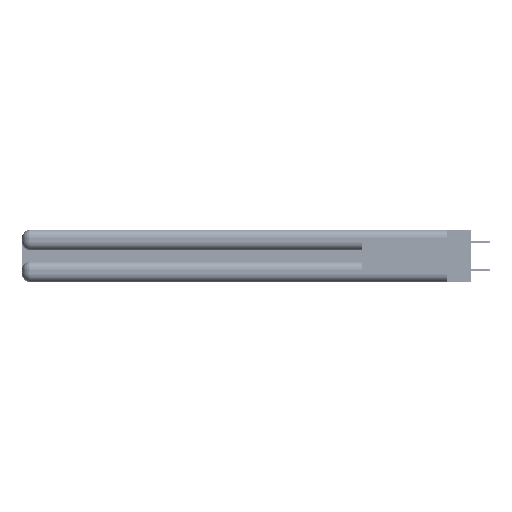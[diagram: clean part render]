
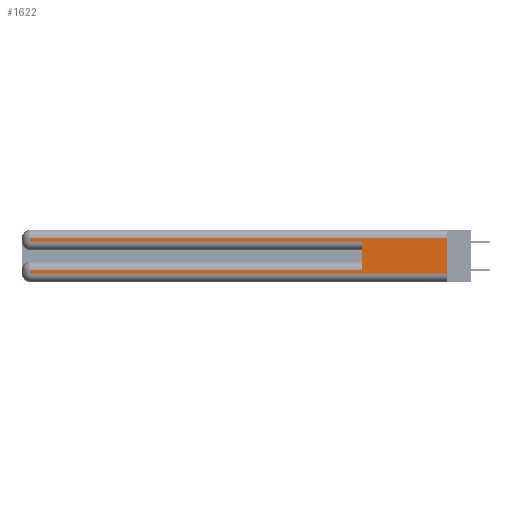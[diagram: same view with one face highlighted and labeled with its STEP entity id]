
A CAD part, left-side view. The second image highlights one B-rep face of the part: STEP entity #1622.
In plain terms, the highlighted planar face has unit normal (-1, 0, 0).
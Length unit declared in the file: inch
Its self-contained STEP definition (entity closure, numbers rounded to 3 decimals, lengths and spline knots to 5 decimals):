
#1622 = ADVANCED_FACE ( 'NONE', ( #33654 ), #19907, .F. ) ;
#1812 = CARTESIAN_POINT ( 'NONE',  ( 0., 2.94, 0.085 ) ) ;
#1971 = VERTEX_POINT ( 'NONE', #1812 ) ;
#2224 = DIRECTION ( 'NONE',  ( 0., -1., 0. ) ) ;
#2310 = ORIENTED_EDGE ( 'NONE', *, *, #7565, .T. ) ;
#2931 = ORIENTED_EDGE ( 'NONE', *, *, #28584, .F. ) ;
#3333 = CARTESIAN_POINT ( 'NONE',  ( 0., 2.94, 0.06 ) ) ;
#4153 = CARTESIAN_POINT ( 'NONE',  ( 0., 0.6, 0.085 ) ) ;
#4446 = CARTESIAN_POINT ( 'NONE',  ( 0., 0., 0.31 ) ) ;
#5204 = LINE ( 'NONE', #13782, #29299 ) ;
#5914 = ORIENTED_EDGE ( 'NONE', *, *, #37096, .T. ) ;
#6305 = VERTEX_POINT ( 'NONE', #4153 ) ;
#6535 = EDGE_CURVE ( 'NONE', #6305, #12182, #52799, .T. ) ;
#7017 = CARTESIAN_POINT ( 'NONE',  ( 0., 0., 0.37 ) ) ;
#7446 = VERTEX_POINT ( 'NONE', #29371 ) ;
#7565 = EDGE_CURVE ( 'NONE', #7446, #44319, #13025, .T. ) ;
#7586 = DIRECTION ( 'NONE',  ( 0., 0., -1. ) ) ;
#7832 = VECTOR ( 'NONE', #31057, 39.37008 ) ;
#11107 = LINE ( 'NONE', #50042, #44562 ) ;
#12182 = VERTEX_POINT ( 'NONE', #29759 ) ;
#13025 = LINE ( 'NONE', #4446, #52068 ) ;
#13201 = CARTESIAN_POINT ( 'NONE',  ( 0., 0., 0.37 ) ) ;
#13220 = DIRECTION ( 'NONE',  ( 0., -1., 0. ) ) ;
#13572 = CARTESIAN_POINT ( 'NONE',  ( 0., 0.6, 0.145 ) ) ;
#13758 = DIRECTION ( 'NONE',  ( 0., 0., -1. ) ) ;
#13782 = CARTESIAN_POINT ( 'NONE',  ( 0., 0., 0.285 ) ) ;
#13937 = VECTOR ( 'NONE', #32113, 39.37008 ) ;
#14042 = LINE ( 'NONE', #13201, #56431 ) ;
#17269 = DIRECTION ( 'NONE',  ( 0., 1., 0. ) ) ;
#17518 = EDGE_CURVE ( 'NONE', #6305, #1971, #34457, .T. ) ;
#19554 = VERTEX_POINT ( 'NONE', #56099 ) ;
#19907 = PLANE ( 'NONE',  #42341 ) ;
#22164 = ORIENTED_EDGE ( 'NONE', *, *, #17518, .T. ) ;
#24303 = ORIENTED_EDGE ( 'NONE', *, *, #27335, .T. ) ;
#27335 = EDGE_CURVE ( 'NONE', #49348, #43812, #11107, .T. ) ;
#28584 = EDGE_CURVE ( 'NONE', #7446, #43812, #14042, .T. ) ;
#28758 = EDGE_CURVE ( 'NONE', #1971, #49348, #46099, .T. ) ;
#29195 = CARTESIAN_POINT ( 'NONE',  ( 0., 0., 0.06 ) ) ;
#29299 = VECTOR ( 'NONE', #13220, 39.37008 ) ;
#29351 = DIRECTION ( 'NONE',  ( 1., 0., 0. ) ) ;
#29371 = CARTESIAN_POINT ( 'NONE',  ( 0., 0., 0.31 ) ) ;
#29523 = ORIENTED_EDGE ( 'NONE', *, *, #6535, .F. ) ;
#29759 = CARTESIAN_POINT ( 'NONE',  ( 0., 0.6, 0.285 ) ) ;
#31057 = DIRECTION ( 'NONE',  ( 0., 0., 1. ) ) ;
#31973 = ORIENTED_EDGE ( 'NONE', *, *, #45968, .T. ) ;
#32113 = DIRECTION ( 'NONE',  ( 0., 0., -1. ) ) ;
#32628 = CARTESIAN_POINT ( 'NONE',  ( 0., 2.94, 0.37 ) ) ;
#33654 = FACE_OUTER_BOUND ( 'NONE', #52486, .T. ) ;
#34457 = LINE ( 'NONE', #47616, #52898 ) ;
#34524 = VECTOR ( 'NONE', #45809, 39.37008 ) ;
#36418 = CARTESIAN_POINT ( 'NONE',  ( 0., 2.94, 0.37 ) ) ;
#37096 = EDGE_CURVE ( 'NONE', #44319, #19554, #44990, .T. ) ;
#38020 = CARTESIAN_POINT ( 'NONE',  ( 0., 2.94, 0.31 ) ) ;
#42341 = AXIS2_PLACEMENT_3D ( 'NONE', #7017, #29351, #7586 ) ;
#43398 = DIRECTION ( 'NONE',  ( 0., 1., 0. ) ) ;
#43812 = VERTEX_POINT ( 'NONE', #29195 ) ;
#44319 = VERTEX_POINT ( 'NONE', #38020 ) ;
#44562 = VECTOR ( 'NONE', #2224, 39.37008 ) ;
#44990 = LINE ( 'NONE', #36418, #13937 ) ;
#45809 = DIRECTION ( 'NONE',  ( 0., 0., -1. ) ) ;
#45968 = EDGE_CURVE ( 'NONE', #19554, #12182, #5204, .T. ) ;
#46099 = LINE ( 'NONE', #32628, #34524 ) ;
#47616 = CARTESIAN_POINT ( 'NONE',  ( 0., 0., 0.085 ) ) ;
#49348 = VERTEX_POINT ( 'NONE', #3333 ) ;
#50042 = CARTESIAN_POINT ( 'NONE',  ( 0., 0., 0.06 ) ) ;
#52068 = VECTOR ( 'NONE', #43398, 39.37008 ) ;
#52486 = EDGE_LOOP ( 'NONE', ( #2931, #2310, #5914, #31973, #29523, #22164, #54632, #24303 ) ) ;
#52799 = LINE ( 'NONE', #13572, #7832 ) ;
#52898 = VECTOR ( 'NONE', #17269, 39.37008 ) ;
#54632 = ORIENTED_EDGE ( 'NONE', *, *, #28758, .T. ) ;
#56099 = CARTESIAN_POINT ( 'NONE',  ( 0., 2.94, 0.285 ) ) ;
#56431 = VECTOR ( 'NONE', #13758, 39.37008 ) ;
